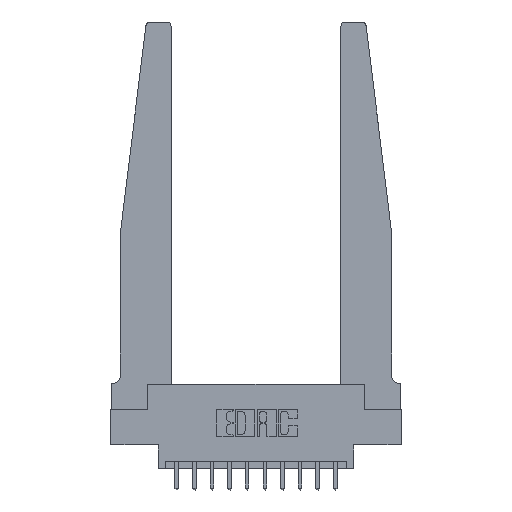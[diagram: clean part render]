
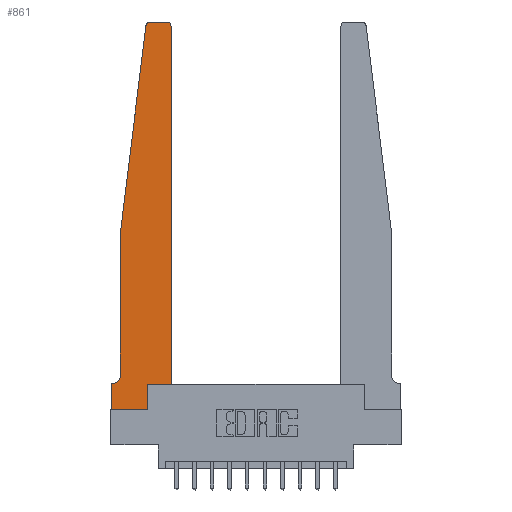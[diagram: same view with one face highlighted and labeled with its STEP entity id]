
A CAD part, top view. The second image highlights one B-rep face of the part: STEP entity #861.
In plain terms, the highlighted planar face has unit normal (0, 0, 1).
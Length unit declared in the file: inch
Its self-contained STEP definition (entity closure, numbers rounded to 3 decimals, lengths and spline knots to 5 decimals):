
#10 = EDGE_CURVE ( 'NONE', #8437, #6518, #1417, .T. ) ;
#62 = AXIS2_PLACEMENT_3D ( 'NONE', #346, #6564, #5330 ) ;
#346 = CARTESIAN_POINT ( 'NONE',  ( 0.015, 0.2375, 0.37 ) ) ;
#368 = FACE_OUTER_BOUND ( 'NONE', #11192, .T. ) ;
#424 = DIRECTION ( 'NONE',  ( 0., 1., 0. ) ) ;
#615 = ORIENTED_EDGE ( 'NONE', *, *, #3702, .T. ) ;
#861 = ADVANCED_FACE ( 'NONE', ( #368 ), #11669, .T. ) ;
#950 = VECTOR ( 'NONE', #4699, 39.37008 ) ;
#1090 = LINE ( 'NONE', #9685, #5501 ) ;
#1227 = ORIENTED_EDGE ( 'NONE', *, *, #6930, .T. ) ;
#1297 = VECTOR ( 'NONE', #15325, 39.37008 ) ;
#1315 = ORIENTED_EDGE ( 'NONE', *, *, #13476, .T. ) ;
#1348 = EDGE_CURVE ( 'NONE', #11583, #5339, #12615, .T. ) ;
#1379 = DIRECTION ( 'NONE',  ( 1., 0., 0. ) ) ;
#1417 = LINE ( 'NONE', #11560, #9242 ) ;
#1494 = LINE ( 'NONE', #6475, #7582 ) ;
#1809 = EDGE_CURVE ( 'NONE', #16147, #11583, #10575, .T. ) ;
#2121 = AXIS2_PLACEMENT_3D ( 'NONE', #4767, #2170, #10852 ) ;
#2160 = CARTESIAN_POINT ( 'NONE',  ( 0., 0.1875, 0.37 ) ) ;
#2170 = DIRECTION ( 'NONE',  ( 0., 0., 1. ) ) ;
#2325 = ORIENTED_EDGE ( 'NONE', *, *, #9796, .T. ) ;
#2347 = EDGE_CURVE ( 'NONE', #6518, #7970, #1494, .T. ) ;
#2500 = EDGE_CURVE ( 'NONE', #5339, #13799, #5587, .T. ) ;
#2576 = AXIS2_PLACEMENT_3D ( 'NONE', #10182, #13999, #10264 ) ;
#3267 = VECTOR ( 'NONE', #10782, 39.37008 ) ;
#3648 = VERTEX_POINT ( 'NONE', #10622 ) ;
#3702 = EDGE_CURVE ( 'NONE', #7970, #3648, #8269, .T. ) ;
#3786 = VERTEX_POINT ( 'NONE', #9871 ) ;
#3880 = DIRECTION ( 'NONE',  ( 1., 0., 0. ) ) ;
#3996 = CARTESIAN_POINT ( 'NONE',  ( 0.425, 0.18, 0.37 ) ) ;
#4359 = CARTESIAN_POINT ( 'NONE',  ( 0.065, 1.25, 0.37 ) ) ;
#4434 = ORIENTED_EDGE ( 'NONE', *, *, #5837, .T. ) ;
#4519 = CARTESIAN_POINT ( 'NONE',  ( 0.065, 1.25, 0.37 ) ) ;
#4699 = DIRECTION ( 'NONE',  ( -1., 0., 0. ) ) ;
#4767 = CARTESIAN_POINT ( 'NONE',  ( 0.395, 2.72, 0.37 ) ) ;
#5330 = DIRECTION ( 'NONE',  ( -1., 0., 0. ) ) ;
#5339 = VERTEX_POINT ( 'NONE', #9362 ) ;
#5350 = CARTESIAN_POINT ( 'NONE',  ( 0., 0.1875, 0.37 ) ) ;
#5501 = VECTOR ( 'NONE', #15981, 39.37008 ) ;
#5587 = LINE ( 'NONE', #10506, #15659 ) ;
#5837 = EDGE_CURVE ( 'NONE', #10228, #8437, #12437, .T. ) ;
#6192 = CARTESIAN_POINT ( 'NONE',  ( 0.27653, 2.75, 0.37 ) ) ;
#6475 = CARTESIAN_POINT ( 'NONE',  ( 0.425, 0.18, 0.37 ) ) ;
#6518 = VERTEX_POINT ( 'NONE', #14014 ) ;
#6564 = DIRECTION ( 'NONE',  ( 0., 0., -1. ) ) ;
#6836 = CIRCLE ( 'NONE', #2121, 0.03 ) ;
#6894 = DIRECTION ( 'NONE',  ( 0., -1., 0. ) ) ;
#6930 = EDGE_CURVE ( 'NONE', #13799, #10228, #14075, .T. ) ;
#7021 = CARTESIAN_POINT ( 'NONE',  ( 0.425, 0.18, 0.37 ) ) ;
#7088 = VECTOR ( 'NONE', #1379, 39.37008 ) ;
#7329 = ORIENTED_EDGE ( 'NONE', *, *, #1348, .T. ) ;
#7582 = VECTOR ( 'NONE', #3880, 39.37008 ) ;
#7749 = CARTESIAN_POINT ( 'NONE',  ( 0., 0., 0.37 ) ) ;
#7970 = VERTEX_POINT ( 'NONE', #3996 ) ;
#8269 = LINE ( 'NONE', #7021, #3267 ) ;
#8410 = LINE ( 'NONE', #12225, #950 ) ;
#8422 = VECTOR ( 'NONE', #6894, 39.37008 ) ;
#8437 = VERTEX_POINT ( 'NONE', #15657 ) ;
#8636 = VERTEX_POINT ( 'NONE', #9603 ) ;
#9134 = DIRECTION ( 'NONE',  ( 0., 0., 1. ) ) ;
#9242 = VECTOR ( 'NONE', #424, 39.37008 ) ;
#9362 = CARTESIAN_POINT ( 'NONE',  ( 0.015, 0.1875, 0.37 ) ) ;
#9564 = ORIENTED_EDGE ( 'NONE', *, *, #1809, .T. ) ;
#9603 = CARTESIAN_POINT ( 'NONE',  ( 0.24675, 2.72367, 0.37 ) ) ;
#9634 = CIRCLE ( 'NONE', #2576, 0.03 ) ;
#9685 = CARTESIAN_POINT ( 'NONE',  ( 0.065, 1.25, 0.37 ) ) ;
#9740 = AXIS2_PLACEMENT_3D ( 'NONE', #5350, #9134, #12970 ) ;
#9796 = EDGE_CURVE ( 'NONE', #8636, #16147, #1090, .T. ) ;
#9871 = CARTESIAN_POINT ( 'NONE',  ( 0.395, 2.75, 0.37 ) ) ;
#9893 = ORIENTED_EDGE ( 'NONE', *, *, #2347, .T. ) ;
#10182 = CARTESIAN_POINT ( 'NONE',  ( 0.27653, 2.72, 0.37 ) ) ;
#10228 = VERTEX_POINT ( 'NONE', #14813 ) ;
#10264 = DIRECTION ( 'NONE',  ( 1., 0., 0. ) ) ;
#10506 = CARTESIAN_POINT ( 'NONE',  ( 0.065, 0.1875, 0.37 ) ) ;
#10575 = LINE ( 'NONE', #4359, #8422 ) ;
#10622 = CARTESIAN_POINT ( 'NONE',  ( 0.425, 2.72, 0.37 ) ) ;
#10782 = DIRECTION ( 'NONE',  ( 0., 1., 0. ) ) ;
#10852 = DIRECTION ( 'NONE',  ( 1., 0., 0. ) ) ;
#11192 = EDGE_LOOP ( 'NONE', ( #15876, #1315, #2325, #9564, #7329, #12910, #1227, #4434, #13423, #9893, #615, #15410 ) ) ;
#11560 = CARTESIAN_POINT ( 'NONE',  ( 0.2605, 0.18, 0.37 ) ) ;
#11583 = VERTEX_POINT ( 'NONE', #13959 ) ;
#11669 = PLANE ( 'NONE',  #9740 ) ;
#12163 = EDGE_CURVE ( 'NONE', #3786, #15032, #8410, .T. ) ;
#12225 = CARTESIAN_POINT ( 'NONE',  ( 0.25, 2.75, 0.37 ) ) ;
#12437 = LINE ( 'NONE', #16183, #7088 ) ;
#12615 = CIRCLE ( 'NONE', #62, 0.05 ) ;
#12910 = ORIENTED_EDGE ( 'NONE', *, *, #2500, .T. ) ;
#12970 = DIRECTION ( 'NONE',  ( 1., 0., 0. ) ) ;
#13027 = DIRECTION ( 'NONE',  ( -1., 0., 0. ) ) ;
#13423 = ORIENTED_EDGE ( 'NONE', *, *, #10, .T. ) ;
#13476 = EDGE_CURVE ( 'NONE', #15032, #8636, #9634, .T. ) ;
#13799 = VERTEX_POINT ( 'NONE', #2160 ) ;
#13959 = CARTESIAN_POINT ( 'NONE',  ( 0.065, 0.2375, 0.37 ) ) ;
#13999 = DIRECTION ( 'NONE',  ( 0., 0., 1. ) ) ;
#14014 = CARTESIAN_POINT ( 'NONE',  ( 0.2605, 0.18, 0.37 ) ) ;
#14075 = LINE ( 'NONE', #7749, #1297 ) ;
#14813 = CARTESIAN_POINT ( 'NONE',  ( 0., 0., 0.37 ) ) ;
#15032 = VERTEX_POINT ( 'NONE', #6192 ) ;
#15325 = DIRECTION ( 'NONE',  ( 0., -1., 0. ) ) ;
#15410 = ORIENTED_EDGE ( 'NONE', *, *, #15785, .T. ) ;
#15657 = CARTESIAN_POINT ( 'NONE',  ( 0.2605, 0., 0.37 ) ) ;
#15659 = VECTOR ( 'NONE', #13027, 39.37008 ) ;
#15785 = EDGE_CURVE ( 'NONE', #3648, #3786, #6836, .T. ) ;
#15876 = ORIENTED_EDGE ( 'NONE', *, *, #12163, .T. ) ;
#15981 = DIRECTION ( 'NONE',  ( -0.122, -0.992, 0. ) ) ;
#16147 = VERTEX_POINT ( 'NONE', #4519 ) ;
#16183 = CARTESIAN_POINT ( 'NONE',  ( 0., 0., 0.37 ) ) ;
